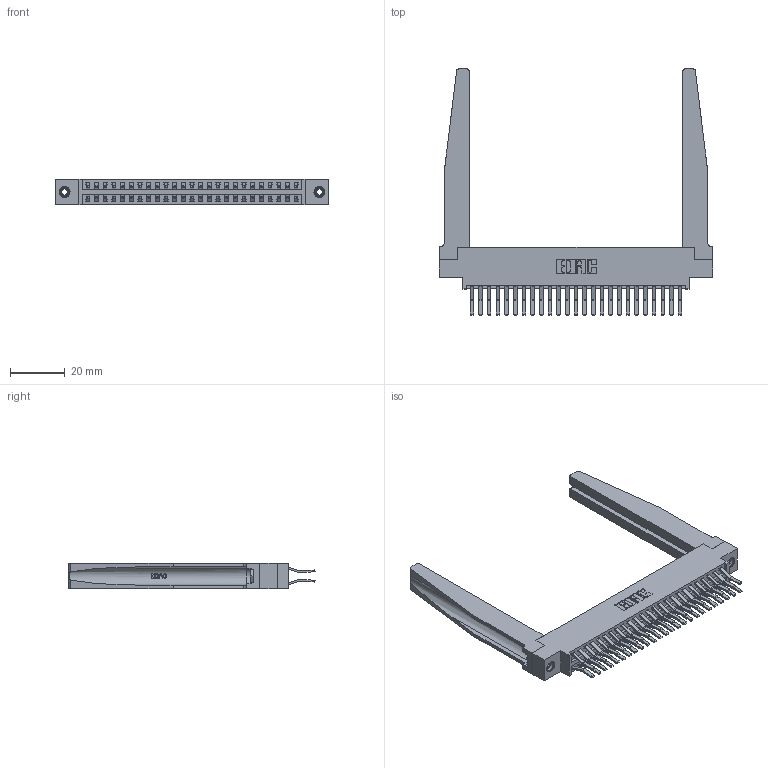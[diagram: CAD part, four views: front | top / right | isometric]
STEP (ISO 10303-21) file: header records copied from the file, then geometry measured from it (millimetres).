
FILE_DESCRIPTION (( 'STEP AP203' ), '1' );
FILE_NAME ('346-050-560-878.STEP', '2022-05-21T00:21:30', ( '' ), ( '' ), 'SwSTEP 2.0', 'SolidWorks 2020', '' );
FILE_SCHEMA (( 'CONFIG_CONTROL_DESIGN' ));
Length unit declared in the file: inch
Products named in the file (5): 345-292-001_560 Tail; 346-220-078_345-220-078; 345-250-001_345-250-001-102; 346 Part_0.170 Offset - 0.156 Dia-TH; 346-050-560-878
Assembly tree (55 placements, depth 2):
  346-050-560-878
    346 Part_0.170 Offset - 0.156 Dia-TH
    345-292-001_560 Tail  x50
    346-220-078_345-220-078  x2
    345-250-001_345-250-001-102  x2
Bounding box: 99.95 x 90.05 x 9.4 mm (x, y, z)
Volume: 16678.1 mm3; surface area: 20787.3 mm2
Topology: 55 solids, 55 shells, 3074 faces, 9035 edges, 5946 vertices
Faces by surface type: plane 1986, cylinder 1036, bspline 36, cone 12, torus 4
Entity records: 23988 total; most frequent: CARTESIAN_POINT 4921, ORIENTED_EDGE 3742, DIRECTION 3377, EDGE_CURVE 1871, LINE 1541, VECTOR 1541, VERTEX_POINT 1240, AXIS2_PLACEMENT_3D 918
